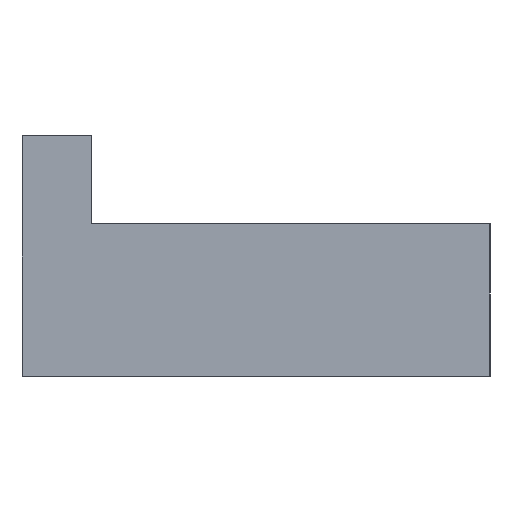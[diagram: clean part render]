
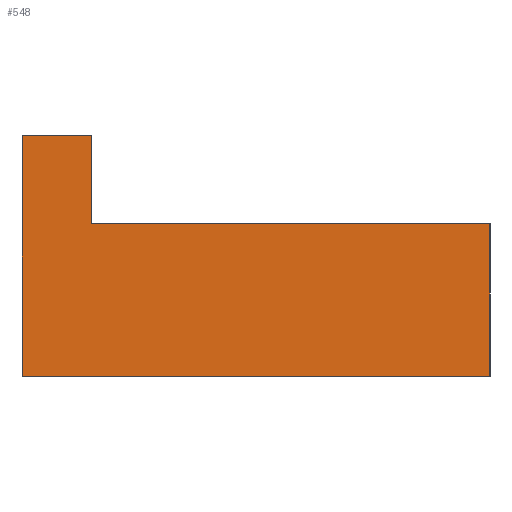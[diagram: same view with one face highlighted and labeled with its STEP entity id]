
A CAD part, left-side view. The second image highlights one B-rep face of the part: STEP entity #548.
In plain terms, the highlighted planar face has unit normal (-1, 0, 0).
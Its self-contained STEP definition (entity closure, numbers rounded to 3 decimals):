
#20=LINE('',#8274,#38);
#23=LINE('',#8926,#41);
#27=LINE('',#8935,#45);
#32=LINE('',#8944,#50);
#35=LINE('',#8949,#53);
#36=LINE('',#8950,#54);
#38=VECTOR('',#620,10.);
#41=VECTOR('',#625,10.);
#45=VECTOR('',#631,10.);
#50=VECTOR('',#638,10.);
#53=VECTOR('',#645,10.);
#54=VECTOR('',#646,10.);
#60=PLANE('',#584);
#80=FACE_OUTER_BOUND('',#100,.T.);
#100=EDGE_LOOP('',(#517,#518,#519,#520,#521,#522));
#244=VERTEX_POINT('',#8271);
#245=VERTEX_POINT('',#8273);
#247=VERTEX_POINT('',#8925);
#249=VERTEX_POINT('',#8931);
#251=VERTEX_POINT('',#8934);
#254=VERTEX_POINT('',#8942);
#326=EDGE_CURVE('',#245,#244,#20,.T.);
#333=EDGE_CURVE('',#247,#244,#23,.T.);
#337=EDGE_CURVE('',#251,#249,#27,.T.);
#342=EDGE_CURVE('',#254,#249,#32,.T.);
#345=EDGE_CURVE('',#245,#254,#35,.T.);
#346=EDGE_CURVE('',#251,#247,#36,.T.);
#517=ORIENTED_EDGE('',*,*,#337,.T.);
#518=ORIENTED_EDGE('',*,*,#342,.F.);
#519=ORIENTED_EDGE('',*,*,#345,.F.);
#520=ORIENTED_EDGE('',*,*,#326,.T.);
#521=ORIENTED_EDGE('',*,*,#333,.F.);
#522=ORIENTED_EDGE('',*,*,#346,.F.);
#548=ADVANCED_FACE('',(#80),#60,.F.);
#584=AXIS2_PLACEMENT_3D('',#8948,#643,#644);
#620=DIRECTION('',(0.,1.,0.));
#625=DIRECTION('',(0.,0.,-1.));
#631=DIRECTION('',(0.,0.,-1.));
#638=DIRECTION('',(0.,1.,0.));
#643=DIRECTION('center_axis',(1.,0.,0.));
#644=DIRECTION('ref_axis',(0.,-1.,0.));
#645=DIRECTION('',(0.,0.,-1.));
#646=DIRECTION('',(0.,-1.,0.));
#8271=CARTESIAN_POINT('',(2.134,0.84,10.036));
#8273=CARTESIAN_POINT('',(2.134,-5.782,10.036));
#8274=CARTESIAN_POINT('',(2.134,0.75,10.036));
#8925=CARTESIAN_POINT('',(2.134,0.84,11.5));
#8926=CARTESIAN_POINT('',(2.134,0.84,10.768));
#8931=CARTESIAN_POINT('',(2.134,2.,7.5));
#8934=CARTESIAN_POINT('',(2.134,2.,11.5));
#8935=CARTESIAN_POINT('',(2.134,2.,9.5));
#8942=CARTESIAN_POINT('',(2.134,-5.782,7.5));
#8944=CARTESIAN_POINT('',(2.134,-6.875,7.5));
#8948=CARTESIAN_POINT('Origin',(2.134,2.5,11.5));
#8949=CARTESIAN_POINT('',(2.134,-5.782,9.5));
#8950=CARTESIAN_POINT('',(2.134,1.34,11.5));
